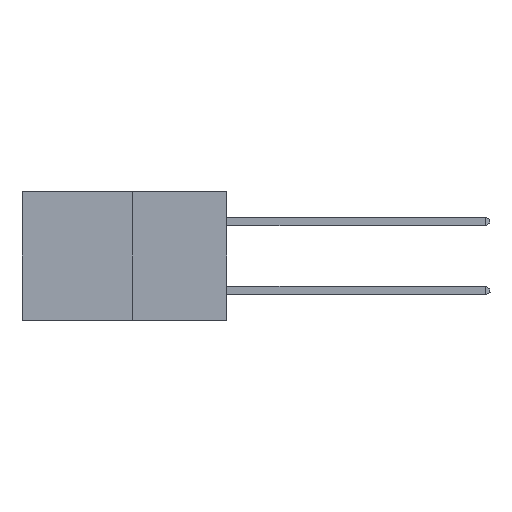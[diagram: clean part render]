
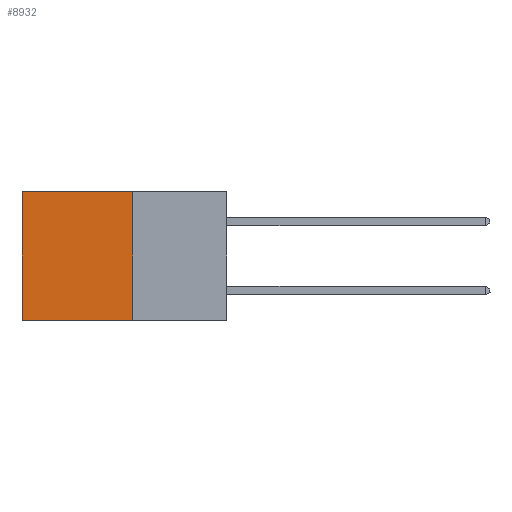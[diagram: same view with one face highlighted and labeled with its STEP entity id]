
A CAD part, left-side view. The second image highlights one B-rep face of the part: STEP entity #8932.
In plain terms, the highlighted planar face has unit normal (-1, 0, 0).
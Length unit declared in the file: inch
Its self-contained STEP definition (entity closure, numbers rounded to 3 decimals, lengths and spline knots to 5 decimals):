
#126 = DIRECTION ( 'NONE',  ( 0., 0., -1. ) ) ;
#1514 = DIRECTION ( 'NONE',  ( 0., 1., 0. ) ) ;
#2347 = CARTESIAN_POINT ( 'NONE',  ( 0.277, 0.27, 0. ) ) ;
#2617 = VECTOR ( 'NONE', #9234, 39.37008 ) ;
#2629 = CARTESIAN_POINT ( 'NONE',  ( 0.277, 0.59, 0. ) ) ;
#2808 = CARTESIAN_POINT ( 'NONE',  ( 0.277, 0.27, -0.37 ) ) ;
#3463 = LINE ( 'NONE', #9894, #6524 ) ;
#3582 = ORIENTED_EDGE ( 'NONE', *, *, #15523, .T. ) ;
#4350 = CARTESIAN_POINT ( 'NONE',  ( 0.277, 0.27, -0.37 ) ) ;
#5267 = ORIENTED_EDGE ( 'NONE', *, *, #13886, .T. ) ;
#5789 = ORIENTED_EDGE ( 'NONE', *, *, #12901, .F. ) ;
#5818 = LINE ( 'NONE', #15107, #15898 ) ;
#5906 = DIRECTION ( 'NONE',  ( 0., 0., -1. ) ) ;
#6074 = LINE ( 'NONE', #10499, #2617 ) ;
#6524 = VECTOR ( 'NONE', #11208, 39.37008 ) ;
#6627 = PLANE ( 'NONE',  #14785 ) ;
#7942 = DIRECTION ( 'NONE',  ( 1., 0., 0. ) ) ;
#8932 = ADVANCED_FACE ( 'NONE', ( #11452 ), #6627, .F. ) ;
#9234 = DIRECTION ( 'NONE',  ( 0., 1., 0. ) ) ;
#9243 = EDGE_LOOP ( 'NONE', ( #3582, #13103, #5789, #5267 ) ) ;
#9258 = VERTEX_POINT ( 'NONE', #2347 ) ;
#9641 = VERTEX_POINT ( 'NONE', #13609 ) ;
#9724 = VECTOR ( 'NONE', #1514, 39.37008 ) ;
#9894 = CARTESIAN_POINT ( 'NONE',  ( 0.277, 0.27, -0.37 ) ) ;
#10499 = CARTESIAN_POINT ( 'NONE',  ( 0.277, 0.27, 0. ) ) ;
#11064 = VERTEX_POINT ( 'NONE', #2629 ) ;
#11208 = DIRECTION ( 'NONE',  ( 0., 0., -1. ) ) ;
#11452 = FACE_OUTER_BOUND ( 'NONE', #9243, .T. ) ;
#12730 = VERTEX_POINT ( 'NONE', #4350 ) ;
#12901 = EDGE_CURVE ( 'NONE', #9258, #12730, #3463, .T. ) ;
#13103 = ORIENTED_EDGE ( 'NONE', *, *, #16643, .F. ) ;
#13609 = CARTESIAN_POINT ( 'NONE',  ( 0.277, 0.59, -0.37 ) ) ;
#13621 = LINE ( 'NONE', #2808, #9724 ) ;
#13886 = EDGE_CURVE ( 'NONE', #9258, #11064, #6074, .T. ) ;
#14489 = CARTESIAN_POINT ( 'NONE',  ( 0.277, 0.27, -0.37 ) ) ;
#14785 = AXIS2_PLACEMENT_3D ( 'NONE', #14489, #7942, #126 ) ;
#15107 = CARTESIAN_POINT ( 'NONE',  ( 0.277, 0.59, -0.37 ) ) ;
#15523 = EDGE_CURVE ( 'NONE', #11064, #9641, #5818, .T. ) ;
#15898 = VECTOR ( 'NONE', #5906, 39.37008 ) ;
#16643 = EDGE_CURVE ( 'NONE', #12730, #9641, #13621, .T. ) ;
